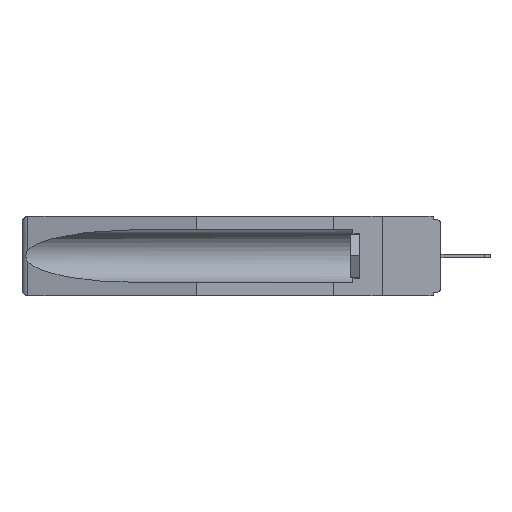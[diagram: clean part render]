
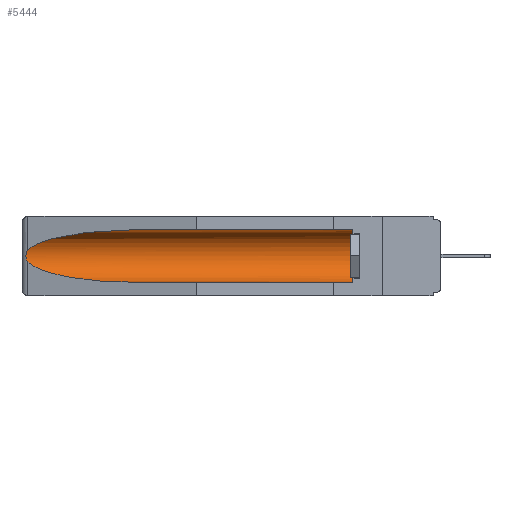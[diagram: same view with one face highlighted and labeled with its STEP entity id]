
A CAD part, left-side view. The second image highlights one B-rep face of the part: STEP entity #5444.
In plain terms, the highlighted cylindrical face has radius 2.857 mm (diameter 5.715 mm), a partial arc.
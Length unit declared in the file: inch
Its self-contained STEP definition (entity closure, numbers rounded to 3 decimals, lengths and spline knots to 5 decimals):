
#113 = VERTEX_POINT ( 'NONE', #20540 ) ;
#1237 = CARTESIAN_POINT ( 'NONE',  ( 0.155, 1.07973, -0.059 ) ) ;
#1299 = CARTESIAN_POINT ( 'NONE',  ( 0.26537, 1.52718, -0.14972 ) ) ;
#1413 = DIRECTION ( 'NONE',  ( 0., 0., 1. ) ) ;
#1750 = DIRECTION ( 'NONE',  ( 0., 1., 0. ) ) ;
#1759 = EDGE_LOOP ( 'NONE', ( #18892, #14752, #6441, #13953, #4937, #17164 ) ) ;
#2287 = FACE_OUTER_BOUND ( 'NONE', #1759, .T. ) ;
#2408 =( BOUNDED_CURVE ( )  B_SPLINE_CURVE ( 3, ( #1237, #10877, #15689, #6096 ),
 .UNSPECIFIED., .F., .F. ) 
 B_SPLINE_CURVE_WITH_KNOTS ( ( 4, 4 ),
 ( 4.71239, 6.08839 ),
 .UNSPECIFIED. ) 
 CURVE ( )  GEOMETRIC_REPRESENTATION_ITEM ( )  RATIONAL_B_SPLINE_CURVE ( ( 1., 0.848, 0.848, 1. ) ) 
 REPRESENTATION_ITEM ( '' )  );
#2599 = VERTEX_POINT ( 'NONE', #6175 ) ;
#2839 = LINE ( 'NONE', #4314, #11372 ) ;
#2959 = VERTEX_POINT ( 'NONE', #9457 ) ;
#4064 = EDGE_CURVE ( 'NONE', #2599, #2959, #2839, .T. ) ;
#4314 = CARTESIAN_POINT ( 'NONE',  ( 0.155, -0.30754, -0.059 ) ) ;
#4464 = DIRECTION ( 'NONE',  ( 0., 1., 0. ) ) ;
#4555 = CARTESIAN_POINT ( 'NONE',  ( 0.2673, 1.5327, -0.16383 ) ) ;
#4937 = ORIENTED_EDGE ( 'NONE', *, *, #12845, .T. ) ;
#5444 = ADVANCED_FACE ( 'NONE', ( #2287 ), #18232, .F. ) ;
#5905 = CARTESIAN_POINT ( 'NONE',  ( 0.155, 1.07973, -0.284 ) ) ;
#6096 = CARTESIAN_POINT ( 'NONE',  ( 0.26537, 1.52718, -0.14972 ) ) ;
#6152 = CARTESIAN_POINT ( 'NONE',  ( 0.2675, 1.53308, -0.17534 ) ) ;
#6175 = CARTESIAN_POINT ( 'NONE',  ( 0.155, 0.126, -0.059 ) ) ;
#6441 = ORIENTED_EDGE ( 'NONE', *, *, #14499, .T. ) ;
#6733 = AXIS2_PLACEMENT_3D ( 'NONE', #20500, #11043, #1413 ) ;
#7094 = B_SPLINE_CURVE_WITH_KNOTS ( 'NONE', 3,
 ( #1299, #10938, #14144, #4555, #15746, #6152, #17316, #7764, #18884, #9405 ),
 .UNSPECIFIED., .F., .F.,
 ( 4, 2, 2, 2, 4 ),
 ( 0., 0.00029, 0.00058, 0.00087, 0.00117 ),
 .UNSPECIFIED. ) ;
#7680 = CARTESIAN_POINT ( 'NONE',  ( 0.155, -0.30754, -0.1715 ) ) ;
#7748 = DIRECTION ( 'NONE',  ( 0., 0., 1. ) ) ;
#7764 = CARTESIAN_POINT ( 'NONE',  ( 0.26655, 1.53094, -0.18657 ) ) ;
#9085 = CARTESIAN_POINT ( 'NONE',  ( 0.26537, 1.52718, -0.19328 ) ) ;
#9405 = CARTESIAN_POINT ( 'NONE',  ( 0.26537, 1.52718, -0.19328 ) ) ;
#9436 = VECTOR ( 'NONE', #1750, 39.37008 ) ;
#9457 = CARTESIAN_POINT ( 'NONE',  ( 0.155, 1.07973, -0.059 ) ) ;
#9772 = CARTESIAN_POINT ( 'NONE',  ( 0.155, -0.30754, -0.284 ) ) ;
#9949 = LINE ( 'NONE', #9772, #9436 ) ;
#10535 = VERTEX_POINT ( 'NONE', #14571 ) ;
#10692 = CARTESIAN_POINT ( 'NONE',  ( 0.25451, 1.48313, -0.24835 ) ) ;
#10877 = CARTESIAN_POINT ( 'NONE',  ( 0.21114, 1.30732, -0.059 ) ) ;
#10938 = CARTESIAN_POINT ( 'NONE',  ( 0.26597, 1.52961, -0.15275 ) ) ;
#11043 = DIRECTION ( 'NONE',  ( 0., -1., 0. ) ) ;
#11372 = VECTOR ( 'NONE', #15511, 39.37008 ) ;
#11626 = EDGE_CURVE ( 'NONE', #2959, #13002, #2408, .T. ) ;
#11857 = CIRCLE ( 'NONE', #6733, 0.1125 ) ;
#12845 = EDGE_CURVE ( 'NONE', #113, #2599, #11857, .T. ) ;
#13002 = VERTEX_POINT ( 'NONE', #17761 ) ;
#13944 = EDGE_CURVE ( 'NONE', #13002, #17599, #7094, .T. ) ;
#13953 = ORIENTED_EDGE ( 'NONE', *, *, #17646, .F. ) ;
#14144 = CARTESIAN_POINT ( 'NONE',  ( 0.26654, 1.53092, -0.15636 ) ) ;
#14499 = EDGE_CURVE ( 'NONE', #17599, #10535, #15022, .T. ) ;
#14571 = CARTESIAN_POINT ( 'NONE',  ( 0.155, 1.07973, -0.284 ) ) ;
#14752 = ORIENTED_EDGE ( 'NONE', *, *, #13944, .T. ) ;
#15022 =( BOUNDED_CURVE ( )  B_SPLINE_CURVE ( 3, ( #9085, #10692, #15527, #5905 ),
 .UNSPECIFIED., .F., .T. ) 
 B_SPLINE_CURVE_WITH_KNOTS ( ( 4, 4 ),
 ( 0.1948, 1.5708 ),
 .UNSPECIFIED. ) 
 CURVE ( )  GEOMETRIC_REPRESENTATION_ITEM ( )  RATIONAL_B_SPLINE_CURVE ( ( 1., 0.848, 0.848, 1. ) ) 
 REPRESENTATION_ITEM ( '' )  );
#15511 = DIRECTION ( 'NONE',  ( 0., 1., 0. ) ) ;
#15527 = CARTESIAN_POINT ( 'NONE',  ( 0.21114, 1.30732, -0.284 ) ) ;
#15689 = CARTESIAN_POINT ( 'NONE',  ( 0.25451, 1.48313, -0.09465 ) ) ;
#15746 = CARTESIAN_POINT ( 'NONE',  ( 0.2675, 1.53308, -0.16763 ) ) ;
#17164 = ORIENTED_EDGE ( 'NONE', *, *, #4064, .T. ) ;
#17316 = CARTESIAN_POINT ( 'NONE',  ( 0.2673, 1.53269, -0.17917 ) ) ;
#17599 = VERTEX_POINT ( 'NONE', #19167 ) ;
#17646 = EDGE_CURVE ( 'NONE', #113, #10535, #9949, .T. ) ;
#17761 = CARTESIAN_POINT ( 'NONE',  ( 0.26537, 1.52718, -0.14972 ) ) ;
#18232 = CYLINDRICAL_SURFACE ( 'NONE', #19137, 0.1125 ) ;
#18884 = CARTESIAN_POINT ( 'NONE',  ( 0.26597, 1.5296, -0.19026 ) ) ;
#18892 = ORIENTED_EDGE ( 'NONE', *, *, #11626, .T. ) ;
#19137 = AXIS2_PLACEMENT_3D ( 'NONE', #7680, #4464, #7748 ) ;
#19167 = CARTESIAN_POINT ( 'NONE',  ( 0.26537, 1.52718, -0.19328 ) ) ;
#20500 = CARTESIAN_POINT ( 'NONE',  ( 0.155, 0.126, -0.1715 ) ) ;
#20540 = CARTESIAN_POINT ( 'NONE',  ( 0.155, 0.126, -0.284 ) ) ;
